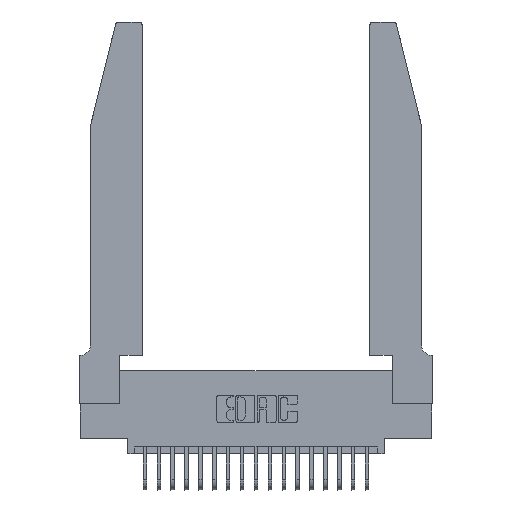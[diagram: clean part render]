
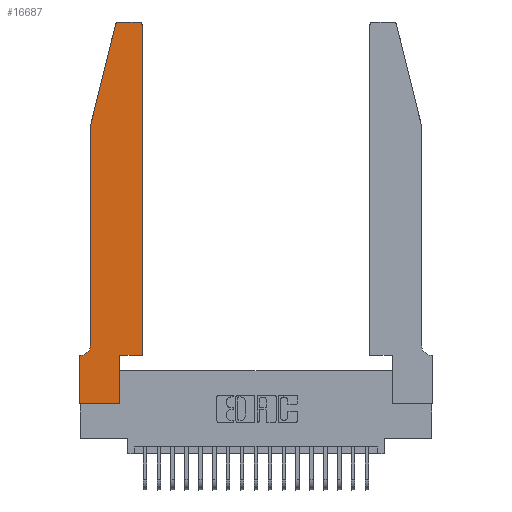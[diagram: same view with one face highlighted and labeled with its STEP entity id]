
A CAD part, top view. The second image highlights one B-rep face of the part: STEP entity #16687.
In plain terms, the highlighted planar face has unit normal (0, 0, 1).
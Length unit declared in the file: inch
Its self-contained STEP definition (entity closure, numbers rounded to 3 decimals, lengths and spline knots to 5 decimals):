
#176 = DIRECTION ( 'NONE',  ( 1., 0., 0. ) ) ;
#283 = VERTEX_POINT ( 'NONE', #12202 ) ;
#601 = ORIENTED_EDGE ( 'NONE', *, *, #12403, .T. ) ;
#880 = DIRECTION ( 'NONE',  ( 0., 1., 0. ) ) ;
#971 = ORIENTED_EDGE ( 'NONE', *, *, #7081, .T. ) ;
#1072 = VERTEX_POINT ( 'NONE', #22850 ) ;
#1105 = DIRECTION ( 'NONE',  ( 0., 0., 1. ) ) ;
#1317 = LINE ( 'NONE', #11352, #10418 ) ;
#1606 = VECTOR ( 'NONE', #4768, 39.37008 ) ;
#1946 = VERTEX_POINT ( 'NONE', #6648 ) ;
#2272 = VERTEX_POINT ( 'NONE', #18163 ) ;
#2479 = AXIS2_PLACEMENT_3D ( 'NONE', #10594, #23005, #12383 ) ;
#2587 = CIRCLE ( 'NONE', #4630, 0.03 ) ;
#2695 = VECTOR ( 'NONE', #18441, 39.37008 ) ;
#2912 = CARTESIAN_POINT ( 'NONE',  ( 0.2865, 0.35, 0.37 ) ) ;
#3224 = VERTEX_POINT ( 'NONE', #15398 ) ;
#3234 = CARTESIAN_POINT ( 'NONE',  ( 0.0755, 0.35, 0.37 ) ) ;
#3875 = EDGE_CURVE ( 'NONE', #15605, #7438, #22872, .T. ) ;
#4318 = CARTESIAN_POINT ( 'NONE',  ( 0.0055, 0.35, 0.37 ) ) ;
#4365 = LINE ( 'NONE', #22228, #17534 ) ;
#4585 = CARTESIAN_POINT ( 'NONE',  ( 0.0755, 2., 0.37 ) ) ;
#4630 = AXIS2_PLACEMENT_3D ( 'NONE', #8556, #20969, #10344 ) ;
#4768 = DIRECTION ( 'NONE',  ( 0., 1., 0. ) ) ;
#5095 = DIRECTION ( 'NONE',  ( -1., 0., 0. ) ) ;
#5424 = CIRCLE ( 'NONE', #2479, 0.07 ) ;
#5841 = CARTESIAN_POINT ( 'NONE',  ( 0.0755, 2., 0.37 ) ) ;
#6039 = LINE ( 'NONE', #17693, #23257 ) ;
#6442 = AXIS2_PLACEMENT_3D ( 'NONE', #15478, #1105, #13781 ) ;
#6648 = CARTESIAN_POINT ( 'NONE',  ( 0.25487, 2.72718, 0.37 ) ) ;
#6915 = EDGE_CURVE ( 'NONE', #3224, #1072, #17035, .T. ) ;
#7081 = EDGE_CURVE ( 'NONE', #283, #21425, #19477, .T. ) ;
#7438 = VERTEX_POINT ( 'NONE', #12832 ) ;
#8131 = VECTOR ( 'NONE', #16538, 39.37008 ) ;
#8556 = CARTESIAN_POINT ( 'NONE',  ( 0.4205, 2.72, 0.37 ) ) ;
#9092 = CARTESIAN_POINT ( 'NONE',  ( 0.2865, 0.35, 0.37 ) ) ;
#9133 = EDGE_CURVE ( 'NONE', #22002, #2272, #6039, .T. ) ;
#10018 = ORIENTED_EDGE ( 'NONE', *, *, #15375, .T. ) ;
#10243 = EDGE_LOOP ( 'NONE', ( #18038, #10018, #601, #17248, #12361, #22882, #13440, #20013, #22948, #13202, #971, #14442 ) ) ;
#10344 = DIRECTION ( 'NONE',  ( 1., 0., 0. ) ) ;
#10418 = VECTOR ( 'NONE', #11432, 39.37008 ) ;
#10594 = CARTESIAN_POINT ( 'NONE',  ( 0.0055, 0.42, 0.37 ) ) ;
#10723 = EDGE_CURVE ( 'NONE', #19651, #283, #1317, .T. ) ;
#10890 = EDGE_CURVE ( 'NONE', #2272, #19651, #16002, .T. ) ;
#11065 = DIRECTION ( 'NONE',  ( 0., 0., 1. ) ) ;
#11352 = CARTESIAN_POINT ( 'NONE',  ( 0.4505, 0.35, 0.37 ) ) ;
#11432 = DIRECTION ( 'NONE',  ( 1., 0., 0. ) ) ;
#11465 = LINE ( 'NONE', #3234, #20350 ) ;
#11597 = FACE_OUTER_BOUND ( 'NONE', #10243, .T. ) ;
#11957 = VERTEX_POINT ( 'NONE', #20679 ) ;
#12202 = CARTESIAN_POINT ( 'NONE',  ( 0.4505, 0.35, 0.37 ) ) ;
#12361 = ORIENTED_EDGE ( 'NONE', *, *, #17951, .T. ) ;
#12383 = DIRECTION ( 'NONE',  ( -1., 0., 0. ) ) ;
#12403 = EDGE_CURVE ( 'NONE', #1946, #15605, #12876, .T. ) ;
#12681 = EDGE_CURVE ( 'NONE', #15547, #11957, #11465, .T. ) ;
#12832 = CARTESIAN_POINT ( 'NONE',  ( 0.0755, 0.42, 0.37 ) ) ;
#12876 = LINE ( 'NONE', #5841, #8131 ) ;
#13202 = ORIENTED_EDGE ( 'NONE', *, *, #10723, .T. ) ;
#13285 = CARTESIAN_POINT ( 'NONE',  ( 0., 0., 0.37 ) ) ;
#13440 = ORIENTED_EDGE ( 'NONE', *, *, #15591, .T. ) ;
#13447 = VECTOR ( 'NONE', #22491, 39.37008 ) ;
#13781 = DIRECTION ( 'NONE',  ( 1., 0., 0. ) ) ;
#14442 = ORIENTED_EDGE ( 'NONE', *, *, #21635, .T. ) ;
#15206 = DIRECTION ( 'NONE',  ( 0., -1., 0. ) ) ;
#15375 = EDGE_CURVE ( 'NONE', #1072, #1946, #16715, .T. ) ;
#15398 = CARTESIAN_POINT ( 'NONE',  ( 0.4205, 2.75, 0.37 ) ) ;
#15478 = CARTESIAN_POINT ( 'NONE',  ( 0., 0.35, 0.37 ) ) ;
#15547 = VERTEX_POINT ( 'NONE', #4318 ) ;
#15591 = EDGE_CURVE ( 'NONE', #11957, #22002, #4365, .T. ) ;
#15605 = VERTEX_POINT ( 'NONE', #20451 ) ;
#16002 = LINE ( 'NONE', #2912, #1606 ) ;
#16538 = DIRECTION ( 'NONE',  ( -0.239, -0.971, 0. ) ) ;
#16687 = ADVANCED_FACE ( 'NONE', ( #11597 ), #22596, .T. ) ;
#16697 = CARTESIAN_POINT ( 'NONE',  ( 0.2605, 2.75, 0.37 ) ) ;
#16715 = CIRCLE ( 'NONE', #18206, 0.03 ) ;
#17035 = LINE ( 'NONE', #16697, #2695 ) ;
#17248 = ORIENTED_EDGE ( 'NONE', *, *, #3875, .T. ) ;
#17534 = VECTOR ( 'NONE', #15206, 39.37008 ) ;
#17693 = CARTESIAN_POINT ( 'NONE',  ( 0., 0., 0.37 ) ) ;
#17951 = EDGE_CURVE ( 'NONE', #7438, #15547, #5424, .T. ) ;
#18038 = ORIENTED_EDGE ( 'NONE', *, *, #6915, .T. ) ;
#18163 = CARTESIAN_POINT ( 'NONE',  ( 0.2865, 0., 0.37 ) ) ;
#18206 = AXIS2_PLACEMENT_3D ( 'NONE', #21698, #11065, #176 ) ;
#18441 = DIRECTION ( 'NONE',  ( -1., 0., 0. ) ) ;
#19428 = DIRECTION ( 'NONE',  ( 1., 0., 0. ) ) ;
#19477 = LINE ( 'NONE', #20593, #23089 ) ;
#19651 = VERTEX_POINT ( 'NONE', #9092 ) ;
#20013 = ORIENTED_EDGE ( 'NONE', *, *, #9133, .T. ) ;
#20350 = VECTOR ( 'NONE', #5095, 39.37008 ) ;
#20451 = CARTESIAN_POINT ( 'NONE',  ( 0.0755, 2., 0.37 ) ) ;
#20593 = CARTESIAN_POINT ( 'NONE',  ( 0.4505, 0.35, 0.37 ) ) ;
#20679 = CARTESIAN_POINT ( 'NONE',  ( 0., 0.35, 0.37 ) ) ;
#20969 = DIRECTION ( 'NONE',  ( 0., 0., 1. ) ) ;
#21425 = VERTEX_POINT ( 'NONE', #22896 ) ;
#21635 = EDGE_CURVE ( 'NONE', #21425, #3224, #2587, .T. ) ;
#21698 = CARTESIAN_POINT ( 'NONE',  ( 0.284, 2.72, 0.37 ) ) ;
#22002 = VERTEX_POINT ( 'NONE', #13285 ) ;
#22228 = CARTESIAN_POINT ( 'NONE',  ( 0., 0., 0.37 ) ) ;
#22491 = DIRECTION ( 'NONE',  ( 0., -1., 0. ) ) ;
#22596 = PLANE ( 'NONE',  #6442 ) ;
#22850 = CARTESIAN_POINT ( 'NONE',  ( 0.284, 2.75, 0.37 ) ) ;
#22872 = LINE ( 'NONE', #4585, #13447 ) ;
#22882 = ORIENTED_EDGE ( 'NONE', *, *, #12681, .T. ) ;
#22896 = CARTESIAN_POINT ( 'NONE',  ( 0.4505, 2.72, 0.37 ) ) ;
#22948 = ORIENTED_EDGE ( 'NONE', *, *, #10890, .T. ) ;
#23005 = DIRECTION ( 'NONE',  ( 0., 0., -1. ) ) ;
#23089 = VECTOR ( 'NONE', #880, 39.37008 ) ;
#23257 = VECTOR ( 'NONE', #19428, 39.37008 ) ;
